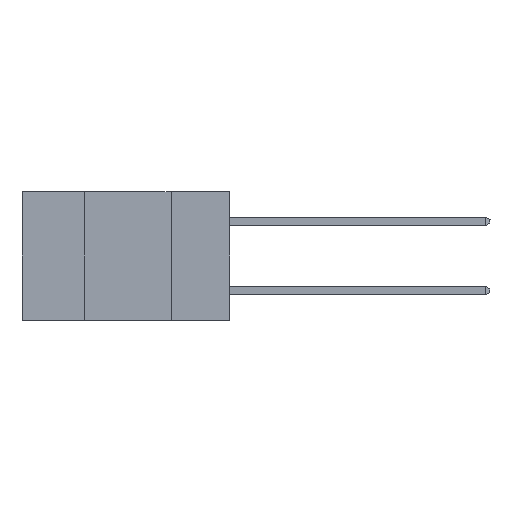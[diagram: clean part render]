
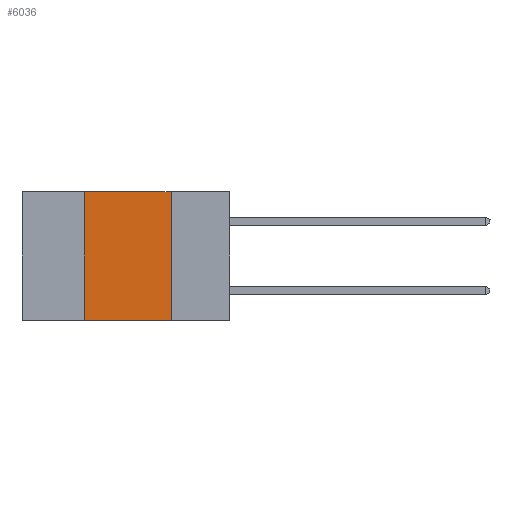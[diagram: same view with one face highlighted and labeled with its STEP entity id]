
A CAD part, left-side view. The second image highlights one B-rep face of the part: STEP entity #6036.
In plain terms, the highlighted planar face has unit normal (-1, 0, 0).
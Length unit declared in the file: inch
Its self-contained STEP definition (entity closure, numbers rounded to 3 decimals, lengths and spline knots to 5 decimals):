
#292 = ORIENTED_EDGE ( 'NONE', *, *, #845, .F. ) ;
#845 = EDGE_CURVE ( 'NONE', #10781, #1551, #6722, .T. ) ;
#1120 = DIRECTION ( 'NONE',  ( 1., 0., 0. ) ) ;
#1489 = VECTOR ( 'NONE', #4814, 39.37008 ) ;
#1551 = VERTEX_POINT ( 'NONE', #9804 ) ;
#2065 = CARTESIAN_POINT ( 'NONE',  ( 0., 0.42, -0.37 ) ) ;
#2464 = VECTOR ( 'NONE', #2602, 39.37008 ) ;
#2602 = DIRECTION ( 'NONE',  ( 0., -1., 0. ) ) ;
#2678 = CARTESIAN_POINT ( 'NONE',  ( 0., 0.6, 0. ) ) ;
#2710 = ORIENTED_EDGE ( 'NONE', *, *, #7842, .T. ) ;
#2879 = CARTESIAN_POINT ( 'NONE',  ( 0., 0.6, 0. ) ) ;
#3962 = LINE ( 'NONE', #4090, #1489 ) ;
#4090 = CARTESIAN_POINT ( 'NONE',  ( 0., 0.17, 0. ) ) ;
#4280 = VERTEX_POINT ( 'NONE', #6870 ) ;
#4437 = DIRECTION ( 'NONE',  ( 0., -1., 0. ) ) ;
#4814 = DIRECTION ( 'NONE',  ( 0., 0., -1. ) ) ;
#4853 = DIRECTION ( 'NONE',  ( 0., 0., 1. ) ) ;
#4895 = VECTOR ( 'NONE', #4437, 39.37008 ) ;
#5026 = ORIENTED_EDGE ( 'NONE', *, *, #8365, .F. ) ;
#5898 = CARTESIAN_POINT ( 'NONE',  ( 0., 0.42, 0. ) ) ;
#6036 = ADVANCED_FACE ( 'NONE', ( #8106 ), #6373, .F. ) ;
#6373 = PLANE ( 'NONE',  #9180 ) ;
#6620 = EDGE_CURVE ( 'NONE', #1551, #4280, #3962, .T. ) ;
#6722 = LINE ( 'NONE', #2678, #2464 ) ;
#6870 = CARTESIAN_POINT ( 'NONE',  ( 0., 0.17, -0.37 ) ) ;
#7223 = VERTEX_POINT ( 'NONE', #2065 ) ;
#7372 = VECTOR ( 'NONE', #4853, 39.37008 ) ;
#7842 = EDGE_CURVE ( 'NONE', #7223, #4280, #10538, .T. ) ;
#8102 = CARTESIAN_POINT ( 'NONE',  ( 0., 0.6, -0.37 ) ) ;
#8106 = FACE_OUTER_BOUND ( 'NONE', #10526, .T. ) ;
#8365 = EDGE_CURVE ( 'NONE', #7223, #10781, #8909, .T. ) ;
#8705 = ORIENTED_EDGE ( 'NONE', *, *, #6620, .F. ) ;
#8909 = LINE ( 'NONE', #9935, #7372 ) ;
#9064 = DIRECTION ( 'NONE',  ( 0., 0., -1. ) ) ;
#9180 = AXIS2_PLACEMENT_3D ( 'NONE', #2879, #1120, #9064 ) ;
#9804 = CARTESIAN_POINT ( 'NONE',  ( 0., 0.17, 0. ) ) ;
#9935 = CARTESIAN_POINT ( 'NONE',  ( 0., 0.42, 0. ) ) ;
#10526 = EDGE_LOOP ( 'NONE', ( #8705, #292, #5026, #2710 ) ) ;
#10538 = LINE ( 'NONE', #8102, #4895 ) ;
#10781 = VERTEX_POINT ( 'NONE', #5898 ) ;
